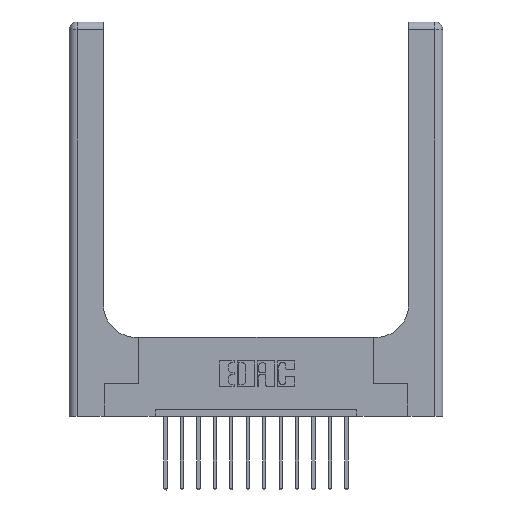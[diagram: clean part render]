
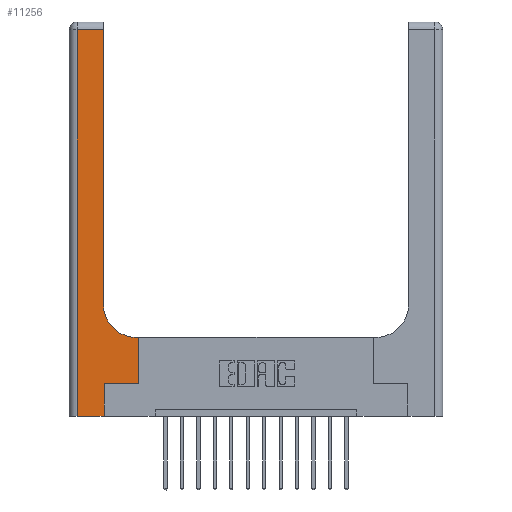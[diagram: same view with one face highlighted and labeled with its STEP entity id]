
A CAD part, top view. The second image highlights one B-rep face of the part: STEP entity #11256.
In plain terms, the highlighted planar face has unit normal (0, 0, 1).
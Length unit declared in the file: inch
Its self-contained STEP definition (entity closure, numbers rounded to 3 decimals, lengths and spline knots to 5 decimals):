
#41 = FACE_OUTER_BOUND ( 'NONE', #4428, .T. ) ;
#122 = CARTESIAN_POINT ( 'NONE',  ( 0.528, 0.6, 0.37 ) ) ;
#150 = ORIENTED_EDGE ( 'NONE', *, *, #11310, .T. ) ;
#223 = DIRECTION ( 'NONE',  ( 1., 0., 0. ) ) ;
#820 = VERTEX_POINT ( 'NONE', #7668 ) ;
#1148 = DIRECTION ( 'NONE',  ( -1., 0., 0. ) ) ;
#1154 = EDGE_CURVE ( 'NONE', #820, #4674, #4245, .T. ) ;
#1347 = CARTESIAN_POINT ( 'NONE',  ( 0.06, 0., 0.37 ) ) ;
#1357 = DIRECTION ( 'NONE',  ( 0., 1., 0. ) ) ;
#1561 = DIRECTION ( 'NONE',  ( 0., 1., 0. ) ) ;
#1885 = CARTESIAN_POINT ( 'NONE',  ( 0.06, 3., 0.37 ) ) ;
#2100 = EDGE_CURVE ( 'NONE', #11967, #16655, #3485, .T. ) ;
#2137 = LINE ( 'NONE', #5226, #7180 ) ;
#2659 = LINE ( 'NONE', #13559, #11705 ) ;
#2836 = CARTESIAN_POINT ( 'NONE',  ( 0.51, 0.85, 0.37 ) ) ;
#3304 = ORIENTED_EDGE ( 'NONE', *, *, #7363, .T. ) ;
#3363 = VECTOR ( 'NONE', #7267, 39.37008 ) ;
#3485 = LINE ( 'NONE', #8831, #5110 ) ;
#3615 = CARTESIAN_POINT ( 'NONE',  ( 0., 3., 0.37 ) ) ;
#3710 = LINE ( 'NONE', #1885, #9531 ) ;
#3936 = DIRECTION ( 'NONE',  ( 1., 0., 0. ) ) ;
#3992 = CARTESIAN_POINT ( 'NONE',  ( 0., 0., 0.37 ) ) ;
#4245 = LINE ( 'NONE', #6280, #16518 ) ;
#4323 = CARTESIAN_POINT ( 'NONE',  ( 0.528, 0.25, 0.37 ) ) ;
#4366 = LINE ( 'NONE', #4669, #3363 ) ;
#4428 = EDGE_LOOP ( 'NONE', ( #5171, #13704, #6045, #4695, #8887, #15726, #10516, #3304, #150 ) ) ;
#4669 = CARTESIAN_POINT ( 'NONE',  ( 0.26, 0.6, 0.37 ) ) ;
#4674 = VERTEX_POINT ( 'NONE', #8021 ) ;
#4695 = ORIENTED_EDGE ( 'NONE', *, *, #10833, .T. ) ;
#5110 = VECTOR ( 'NONE', #1148, 39.37008 ) ;
#5171 = ORIENTED_EDGE ( 'NONE', *, *, #12582, .T. ) ;
#5226 = CARTESIAN_POINT ( 'NONE',  ( 0.265, 0., 0.37 ) ) ;
#6045 = ORIENTED_EDGE ( 'NONE', *, *, #16274, .T. ) ;
#6190 = VERTEX_POINT ( 'NONE', #1347 ) ;
#6211 = DIRECTION ( 'NONE',  ( -1., 0., 0. ) ) ;
#6280 = CARTESIAN_POINT ( 'NONE',  ( 0.265, 0.25, 0.37 ) ) ;
#6336 = LINE ( 'NONE', #3992, #15774 ) ;
#6479 = VERTEX_POINT ( 'NONE', #12159 ) ;
#7180 = VECTOR ( 'NONE', #1357, 39.37008 ) ;
#7267 = DIRECTION ( 'NONE',  ( -1., 0., 0. ) ) ;
#7363 = EDGE_CURVE ( 'NONE', #8675, #14278, #4366, .T. ) ;
#7668 = CARTESIAN_POINT ( 'NONE',  ( 0.265, 0.25, 0.37 ) ) ;
#8021 = CARTESIAN_POINT ( 'NONE',  ( 0.528, 0.25, 0.37 ) ) ;
#8675 = VERTEX_POINT ( 'NONE', #122 ) ;
#8710 = PLANE ( 'NONE',  #15986 ) ;
#8831 = CARTESIAN_POINT ( 'NONE',  ( 0., 2.94, 0.37 ) ) ;
#8887 = ORIENTED_EDGE ( 'NONE', *, *, #9102, .T. ) ;
#9102 = EDGE_CURVE ( 'NONE', #14543, #820, #2137, .T. ) ;
#9531 = VECTOR ( 'NONE', #10644, 39.37008 ) ;
#9960 = DIRECTION ( 'NONE',  ( 0., 0., -1. ) ) ;
#10360 = CARTESIAN_POINT ( 'NONE',  ( 0.06, 2.94, 0.37 ) ) ;
#10516 = ORIENTED_EDGE ( 'NONE', *, *, #13328, .T. ) ;
#10644 = DIRECTION ( 'NONE',  ( 0., -1., 0. ) ) ;
#10833 = EDGE_CURVE ( 'NONE', #6190, #14543, #6336, .T. ) ;
#11076 = DIRECTION ( 'NONE',  ( 0., 1., 0. ) ) ;
#11256 = ADVANCED_FACE ( 'NONE', ( #41 ), #8710, .F. ) ;
#11279 = LINE ( 'NONE', #4323, #12086 ) ;
#11310 = EDGE_CURVE ( 'NONE', #14278, #6479, #15365, .T. ) ;
#11705 = VECTOR ( 'NONE', #11076, 39.37008 ) ;
#11967 = VERTEX_POINT ( 'NONE', #13662 ) ;
#12086 = VECTOR ( 'NONE', #1561, 39.37008 ) ;
#12159 = CARTESIAN_POINT ( 'NONE',  ( 0.26, 0.85, 0.37 ) ) ;
#12582 = EDGE_CURVE ( 'NONE', #6479, #11967, #2659, .T. ) ;
#13328 = EDGE_CURVE ( 'NONE', #4674, #8675, #11279, .T. ) ;
#13559 = CARTESIAN_POINT ( 'NONE',  ( 0.26, 3., 0.37 ) ) ;
#13662 = CARTESIAN_POINT ( 'NONE',  ( 0.26, 2.94, 0.37 ) ) ;
#13704 = ORIENTED_EDGE ( 'NONE', *, *, #2100, .T. ) ;
#14278 = VERTEX_POINT ( 'NONE', #14307 ) ;
#14307 = CARTESIAN_POINT ( 'NONE',  ( 0.51, 0.6, 0.37 ) ) ;
#14543 = VERTEX_POINT ( 'NONE', #16158 ) ;
#15271 = DIRECTION ( 'NONE',  ( 1., 0., 0. ) ) ;
#15365 = CIRCLE ( 'NONE', #16089, 0.25 ) ;
#15642 = DIRECTION ( 'NONE',  ( 0., 0., -1. ) ) ;
#15726 = ORIENTED_EDGE ( 'NONE', *, *, #1154, .T. ) ;
#15774 = VECTOR ( 'NONE', #3936, 39.37008 ) ;
#15986 = AXIS2_PLACEMENT_3D ( 'NONE', #3615, #9960, #6211 ) ;
#16089 = AXIS2_PLACEMENT_3D ( 'NONE', #2836, #15642, #223 ) ;
#16158 = CARTESIAN_POINT ( 'NONE',  ( 0.265, 0., 0.37 ) ) ;
#16274 = EDGE_CURVE ( 'NONE', #16655, #6190, #3710, .T. ) ;
#16518 = VECTOR ( 'NONE', #15271, 39.37008 ) ;
#16655 = VERTEX_POINT ( 'NONE', #10360 ) ;
